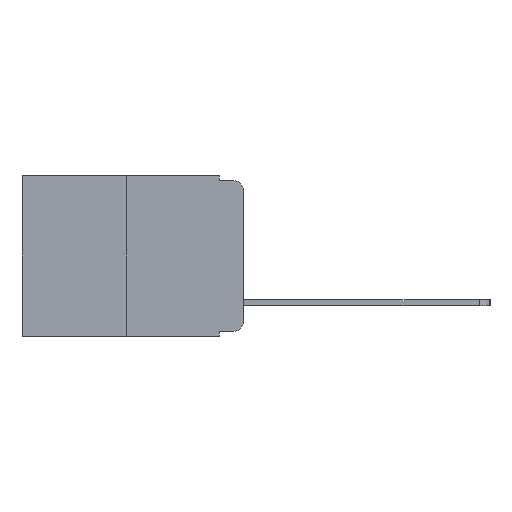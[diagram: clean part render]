
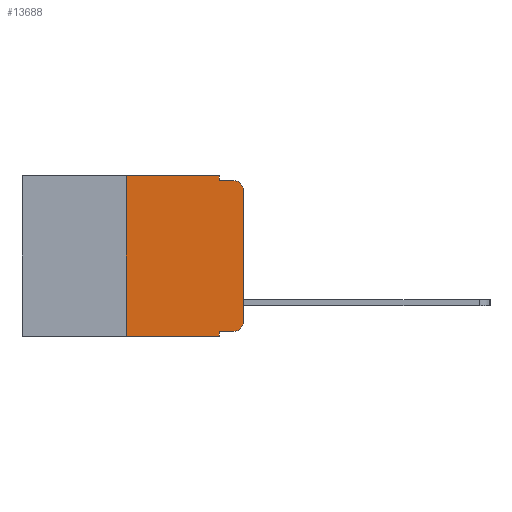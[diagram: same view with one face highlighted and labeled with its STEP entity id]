
A CAD part, left-side view. The second image highlights one B-rep face of the part: STEP entity #13688.
In plain terms, the highlighted planar face has unit normal (-1, 0, 0).
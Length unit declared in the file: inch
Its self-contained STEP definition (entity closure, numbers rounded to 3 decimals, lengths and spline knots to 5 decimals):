
#697 = ORIENTED_EDGE ( 'NONE', *, *, #13641, .F. ) ;
#1416 = CARTESIAN_POINT ( 'NONE',  ( 0., 0.051, -0.333 ) ) ;
#1498 = DIRECTION ( 'NONE',  ( 0., 0., -1. ) ) ;
#1840 = AXIS2_PLACEMENT_3D ( 'NONE', #23265, #12785, #1498 ) ;
#2039 = ORIENTED_EDGE ( 'NONE', *, *, #12455, .T. ) ;
#2833 = VERTEX_POINT ( 'NONE', #5436 ) ;
#2854 = CARTESIAN_POINT ( 'NONE',  ( 0., 0.051, -0.01 ) ) ;
#3340 = ORIENTED_EDGE ( 'NONE', *, *, #11264, .T. ) ;
#4039 = VERTEX_POINT ( 'NONE', #2854 ) ;
#4314 = LINE ( 'NONE', #4437, #14021 ) ;
#4437 = CARTESIAN_POINT ( 'NONE',  ( 0., 0.051, -0.333 ) ) ;
#4758 = VERTEX_POINT ( 'NONE', #15201 ) ;
#5436 = CARTESIAN_POINT ( 'NONE',  ( 0., 0.25, 0. ) ) ;
#5796 = CARTESIAN_POINT ( 'NONE',  ( 0., 0.473, 0. ) ) ;
#5864 = VERTEX_POINT ( 'NONE', #15432 ) ;
#5869 = CARTESIAN_POINT ( 'NONE',  ( 0., 0., -0.03 ) ) ;
#5973 = ORIENTED_EDGE ( 'NONE', *, *, #20674, .T. ) ;
#6069 = LINE ( 'NONE', #14209, #19775 ) ;
#6233 = LINE ( 'NONE', #15299, #15260 ) ;
#6547 = AXIS2_PLACEMENT_3D ( 'NONE', #8846, #21166, #10629 ) ;
#6930 = VECTOR ( 'NONE', #13574, 39.37008 ) ;
#6946 = VERTEX_POINT ( 'NONE', #21586 ) ;
#6952 = PLANE ( 'NONE',  #6547 ) ;
#7062 = ORIENTED_EDGE ( 'NONE', *, *, #18322, .F. ) ;
#7226 = LINE ( 'NONE', #15590, #15610 ) ;
#7453 = ORIENTED_EDGE ( 'NONE', *, *, #19490, .F. ) ;
#7641 = CARTESIAN_POINT ( 'NONE',  ( 0., 0.051, -0.01 ) ) ;
#7737 = DIRECTION ( 'NONE',  ( 0., -1., 0. ) ) ;
#7759 = CARTESIAN_POINT ( 'NONE',  ( 0., 0.051, -0.343 ) ) ;
#7763 = LINE ( 'NONE', #7641, #11997 ) ;
#8676 = CARTESIAN_POINT ( 'NONE',  ( 0., 0.051, 0. ) ) ;
#8846 = CARTESIAN_POINT ( 'NONE',  ( 0., 0.473, 0. ) ) ;
#9050 = VERTEX_POINT ( 'NONE', #7759 ) ;
#9731 = EDGE_CURVE ( 'NONE', #2833, #5864, #22614, .T. ) ;
#10482 = DIRECTION ( 'NONE',  ( 0., 0., -1. ) ) ;
#10629 = DIRECTION ( 'NONE',  ( 0., 0., -1. ) ) ;
#11171 = ORIENTED_EDGE ( 'NONE', *, *, #23017, .T. ) ;
#11264 = EDGE_CURVE ( 'NONE', #4758, #20892, #14366, .T. ) ;
#11460 = DIRECTION ( 'NONE',  ( -1., 0., 0. ) ) ;
#11764 = LINE ( 'NONE', #15316, #6930 ) ;
#11997 = VECTOR ( 'NONE', #21774, 39.37008 ) ;
#12167 = AXIS2_PLACEMENT_3D ( 'NONE', #21950, #11460, #23706 ) ;
#12455 = EDGE_CURVE ( 'NONE', #17973, #4758, #4314, .T. ) ;
#12747 = VERTEX_POINT ( 'NONE', #17741 ) ;
#12785 = DIRECTION ( 'NONE',  ( -1., 0., 0. ) ) ;
#13297 = VECTOR ( 'NONE', #7737, 39.37008 ) ;
#13574 = DIRECTION ( 'NONE',  ( 0., 0., -1. ) ) ;
#13641 = EDGE_CURVE ( 'NONE', #17973, #9050, #19011, .T. ) ;
#13688 = ADVANCED_FACE ( 'NONE', ( #17350 ), #6952, .F. ) ;
#13966 = ORIENTED_EDGE ( 'NONE', *, *, #20989, .T. ) ;
#14021 = VECTOR ( 'NONE', #17057, 39.37008 ) ;
#14209 = CARTESIAN_POINT ( 'NONE',  ( 0., 0.25, 0. ) ) ;
#14366 = CIRCLE ( 'NONE', #12167, 0.02 ) ;
#14898 = VECTOR ( 'NONE', #10482, 39.37008 ) ;
#15201 = CARTESIAN_POINT ( 'NONE',  ( 0., 0.02, -0.333 ) ) ;
#15260 = VECTOR ( 'NONE', #17050, 39.37008 ) ;
#15299 = CARTESIAN_POINT ( 'NONE',  ( 0., 0.473, -0.343 ) ) ;
#15316 = CARTESIAN_POINT ( 'NONE',  ( 0., 0.051, 0. ) ) ;
#15432 = CARTESIAN_POINT ( 'NONE',  ( 0., 0.051, 0. ) ) ;
#15434 = VERTEX_POINT ( 'NONE', #5869 ) ;
#15590 = CARTESIAN_POINT ( 'NONE',  ( 0., 0., 0. ) ) ;
#15610 = VECTOR ( 'NONE', #22470, 39.37008 ) ;
#15649 = ORIENTED_EDGE ( 'NONE', *, *, #17142, .F. ) ;
#16626 = CIRCLE ( 'NONE', #1840, 0.02 ) ;
#17050 = DIRECTION ( 'NONE',  ( 0., -1., 0. ) ) ;
#17057 = DIRECTION ( 'NONE',  ( 0., -1., 0. ) ) ;
#17142 = EDGE_CURVE ( 'NONE', #12747, #2833, #6069, .T. ) ;
#17350 = FACE_OUTER_BOUND ( 'NONE', #17947, .T. ) ;
#17726 = DIRECTION ( 'NONE',  ( 0., 0., 1. ) ) ;
#17741 = CARTESIAN_POINT ( 'NONE',  ( 0., 0.25, -0.343 ) ) ;
#17947 = EDGE_LOOP ( 'NONE', ( #11171, #5973, #7453, #7062, #21942, #15649, #13966, #697, #2039, #3340 ) ) ;
#17973 = VERTEX_POINT ( 'NONE', #1416 ) ;
#18322 = EDGE_CURVE ( 'NONE', #5864, #4039, #11764, .T. ) ;
#19011 = LINE ( 'NONE', #8676, #14898 ) ;
#19490 = EDGE_CURVE ( 'NONE', #4039, #6946, #7763, .T. ) ;
#19775 = VECTOR ( 'NONE', #17726, 39.37008 ) ;
#20353 = CARTESIAN_POINT ( 'NONE',  ( 0., 0., -0.313 ) ) ;
#20674 = EDGE_CURVE ( 'NONE', #15434, #6946, #16626, .T. ) ;
#20892 = VERTEX_POINT ( 'NONE', #20353 ) ;
#20989 = EDGE_CURVE ( 'NONE', #12747, #9050, #6233, .T. ) ;
#21166 = DIRECTION ( 'NONE',  ( 1., 0., 0. ) ) ;
#21586 = CARTESIAN_POINT ( 'NONE',  ( 0., 0.02, -0.01 ) ) ;
#21774 = DIRECTION ( 'NONE',  ( 0., -1., 0. ) ) ;
#21942 = ORIENTED_EDGE ( 'NONE', *, *, #9731, .F. ) ;
#21950 = CARTESIAN_POINT ( 'NONE',  ( 0., 0.02, -0.313 ) ) ;
#22470 = DIRECTION ( 'NONE',  ( 0., 0., 1. ) ) ;
#22614 = LINE ( 'NONE', #5796, #13297 ) ;
#23017 = EDGE_CURVE ( 'NONE', #20892, #15434, #7226, .T. ) ;
#23265 = CARTESIAN_POINT ( 'NONE',  ( 0., 0.02, -0.03 ) ) ;
#23706 = DIRECTION ( 'NONE',  ( 0., 0., -1. ) ) ;
